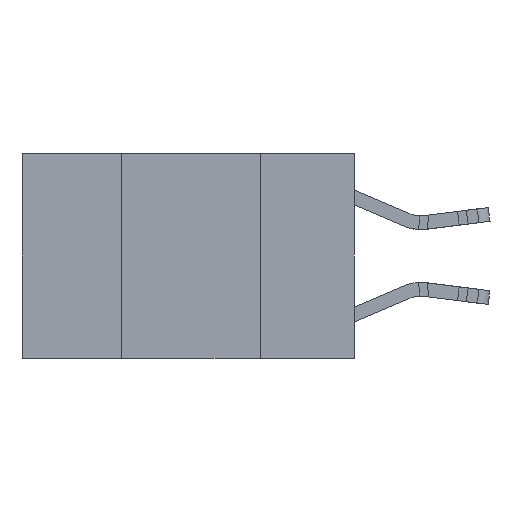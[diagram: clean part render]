
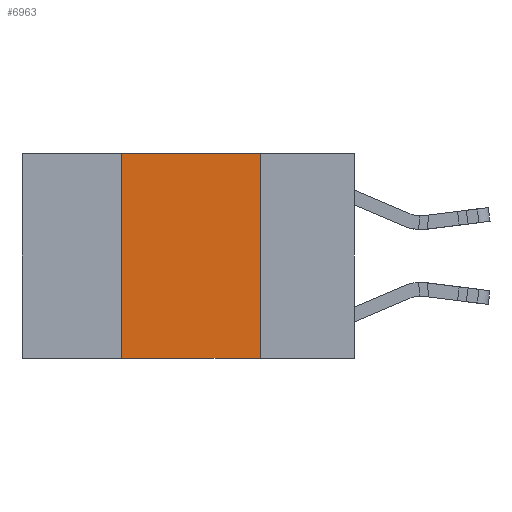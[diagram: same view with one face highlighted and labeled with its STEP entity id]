
A CAD part, left-side view. The second image highlights one B-rep face of the part: STEP entity #6963.
In plain terms, the highlighted planar face has unit normal (-1, 0, 0).
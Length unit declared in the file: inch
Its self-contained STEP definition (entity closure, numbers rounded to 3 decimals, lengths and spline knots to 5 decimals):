
#185 = CARTESIAN_POINT ( 'NONE',  ( 0., 0.17, -0.37 ) ) ;
#557 = CARTESIAN_POINT ( 'NONE',  ( 0., 0.6, 0. ) ) ;
#978 = VECTOR ( 'NONE', #17542, 39.37008 ) ;
#3203 = CARTESIAN_POINT ( 'NONE',  ( 0., 0.17, 0. ) ) ;
#5341 = VERTEX_POINT ( 'NONE', #21364 ) ;
#5439 = DIRECTION ( 'NONE',  ( 0., 0., -1. ) ) ;
#5752 = ORIENTED_EDGE ( 'NONE', *, *, #19740, .F. ) ;
#6196 = VERTEX_POINT ( 'NONE', #185 ) ;
#6740 = DIRECTION ( 'NONE',  ( 0., 0., 1. ) ) ;
#6818 = CARTESIAN_POINT ( 'NONE',  ( 0., 0.42, -0.37 ) ) ;
#6963 = ADVANCED_FACE ( 'NONE', ( #26033 ), #17525, .F. ) ;
#8998 = VERTEX_POINT ( 'NONE', #6818 ) ;
#9254 = AXIS2_PLACEMENT_3D ( 'NONE', #557, #19929, #5439 ) ;
#9563 = LINE ( 'NONE', #3203, #27955 ) ;
#11940 = CARTESIAN_POINT ( 'NONE',  ( 0., 0.6, -0.37 ) ) ;
#12191 = ORIENTED_EDGE ( 'NONE', *, *, #26935, .F. ) ;
#13959 = VECTOR ( 'NONE', #6740, 39.37008 ) ;
#17525 = PLANE ( 'NONE',  #9254 ) ;
#17542 = DIRECTION ( 'NONE',  ( 0., -1., 0. ) ) ;
#19740 = EDGE_CURVE ( 'NONE', #24749, #5341, #21765, .T. ) ;
#19929 = DIRECTION ( 'NONE',  ( 1., 0., 0. ) ) ;
#20046 = CARTESIAN_POINT ( 'NONE',  ( 0., 0.6, 0. ) ) ;
#20710 = VECTOR ( 'NONE', #28702, 39.37008 ) ;
#21364 = CARTESIAN_POINT ( 'NONE',  ( 0., 0.17, 0. ) ) ;
#21765 = LINE ( 'NONE', #20046, #978 ) ;
#23729 = EDGE_CURVE ( 'NONE', #5341, #6196, #9563, .T. ) ;
#24749 = VERTEX_POINT ( 'NONE', #30781 ) ;
#24910 = DIRECTION ( 'NONE',  ( 0., 0., -1. ) ) ;
#25714 = ORIENTED_EDGE ( 'NONE', *, *, #30122, .T. ) ;
#25954 = EDGE_LOOP ( 'NONE', ( #30545, #5752, #12191, #25714 ) ) ;
#25984 = CARTESIAN_POINT ( 'NONE',  ( 0., 0.42, 0. ) ) ;
#26033 = FACE_OUTER_BOUND ( 'NONE', #25954, .T. ) ;
#26288 = LINE ( 'NONE', #11940, #20710 ) ;
#26684 = LINE ( 'NONE', #25984, #13959 ) ;
#26935 = EDGE_CURVE ( 'NONE', #8998, #24749, #26684, .T. ) ;
#27955 = VECTOR ( 'NONE', #24910, 39.37008 ) ;
#28702 = DIRECTION ( 'NONE',  ( 0., -1., 0. ) ) ;
#30122 = EDGE_CURVE ( 'NONE', #8998, #6196, #26288, .T. ) ;
#30545 = ORIENTED_EDGE ( 'NONE', *, *, #23729, .F. ) ;
#30781 = CARTESIAN_POINT ( 'NONE',  ( 0., 0.42, 0. ) ) ;
